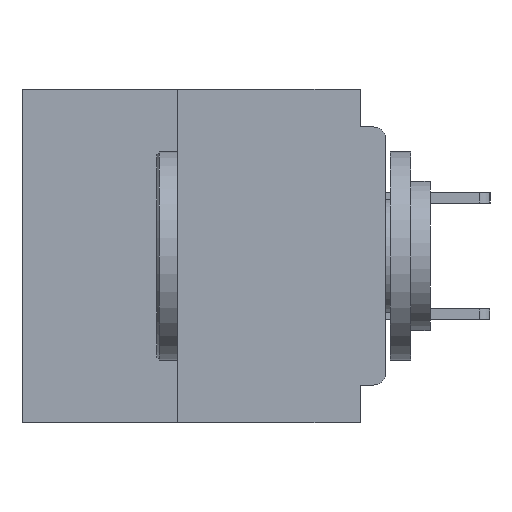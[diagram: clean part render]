
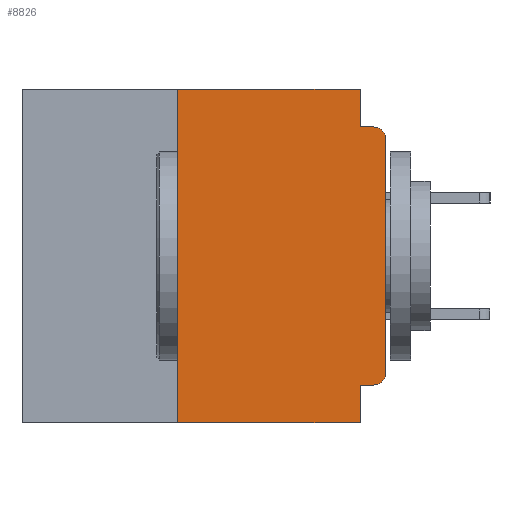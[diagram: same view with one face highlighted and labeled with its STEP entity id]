
A CAD part, left-side view. The second image highlights one B-rep face of the part: STEP entity #8826.
In plain terms, the highlighted planar face has unit normal (-1, 0, 0).
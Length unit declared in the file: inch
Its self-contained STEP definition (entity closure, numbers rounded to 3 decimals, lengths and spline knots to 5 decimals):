
#51 = VERTEX_POINT ( 'NONE', #12054 ) ;
#124 = LINE ( 'NONE', #33664, #1399 ) ;
#156 = FACE_OUTER_BOUND ( 'NONE', #11290, .T. ) ;
#342 = AXIS2_PLACEMENT_3D ( 'NONE', #40303, #16422, #44274 ) ;
#838 = CARTESIAN_POINT ( 'NONE',  ( 0., 0.437, 0. ) ) ;
#1216 = VERTEX_POINT ( 'NONE', #44864 ) ;
#1399 = VECTOR ( 'NONE', #13725, 39.37008 ) ;
#2683 = EDGE_CURVE ( 'NONE', #10931, #44653, #49319, .T. ) ;
#5147 = CARTESIAN_POINT ( 'NONE',  ( 0., 0., 0. ) ) ;
#6038 = VERTEX_POINT ( 'NONE', #50441 ) ;
#7062 = CARTESIAN_POINT ( 'NONE',  ( 0., 0.031, -0.355 ) ) ;
#7773 = CARTESIAN_POINT ( 'NONE',  ( 0., 0.031, -0.045 ) ) ;
#8325 = EDGE_CURVE ( 'NONE', #23445, #51, #45398, .T. ) ;
#8826 = ADVANCED_FACE ( 'NONE', ( #156 ), #36322, .F. ) ;
#9465 = CARTESIAN_POINT ( 'NONE',  ( 0., 0.031, -0.4 ) ) ;
#10931 = VERTEX_POINT ( 'NONE', #7062 ) ;
#11290 = EDGE_LOOP ( 'NONE', ( #17904, #48999, #14149, #24215, #12917, #45977, #40409, #33611, #34852, #19923 ) ) ;
#11738 = CARTESIAN_POINT ( 'NONE',  ( 0., 0.25, -0.4 ) ) ;
#12054 = CARTESIAN_POINT ( 'NONE',  ( 0., 0.015, -0.045 ) ) ;
#12917 = ORIENTED_EDGE ( 'NONE', *, *, #33629, .F. ) ;
#13236 = VECTOR ( 'NONE', #13382, 39.37008 ) ;
#13382 = DIRECTION ( 'NONE',  ( 0., 0., 1. ) ) ;
#13483 = CARTESIAN_POINT ( 'NONE',  ( 0., 0., -0.355 ) ) ;
#13725 = DIRECTION ( 'NONE',  ( 0., -1., 0. ) ) ;
#13757 = DIRECTION ( 'NONE',  ( 0., 0., -1. ) ) ;
#14149 = ORIENTED_EDGE ( 'NONE', *, *, #31255, .F. ) ;
#14887 = LINE ( 'NONE', #11738, #44169 ) ;
#15347 = LINE ( 'NONE', #48682, #50838 ) ;
#15582 = CARTESIAN_POINT ( 'NONE',  ( 0., 0., -0.06 ) ) ;
#16422 = DIRECTION ( 'NONE',  ( 1., 0., 0. ) ) ;
#16811 = CARTESIAN_POINT ( 'NONE',  ( 0., 0.25, -0.4 ) ) ;
#17904 = ORIENTED_EDGE ( 'NONE', *, *, #34433, .T. ) ;
#18618 = CIRCLE ( 'NONE', #23411, 0.015 ) ;
#19085 = VERTEX_POINT ( 'NONE', #39088 ) ;
#19464 = VECTOR ( 'NONE', #29627, 39.37008 ) ;
#19923 = ORIENTED_EDGE ( 'NONE', *, *, #20035, .T. ) ;
#20035 = EDGE_CURVE ( 'NONE', #19085, #1216, #18618, .T. ) ;
#20743 = LINE ( 'NONE', #13483, #19464 ) ;
#21124 = DIRECTION ( 'NONE',  ( 0., -1., 0. ) ) ;
#21280 = DIRECTION ( 'NONE',  ( 0., -1., 0. ) ) ;
#21284 = LINE ( 'NONE', #37686, #31848 ) ;
#21414 = VECTOR ( 'NONE', #35941, 39.37008 ) ;
#21623 = VERTEX_POINT ( 'NONE', #7773 ) ;
#21632 = DIRECTION ( 'NONE',  ( -1., 0., 0. ) ) ;
#22126 = CARTESIAN_POINT ( 'NONE',  ( 0., 0.015, -0.34 ) ) ;
#23411 = AXIS2_PLACEMENT_3D ( 'NONE', #22126, #49857, #26115 ) ;
#23445 = VERTEX_POINT ( 'NONE', #15582 ) ;
#23892 = DIRECTION ( 'NONE',  ( 0., 0., 1. ) ) ;
#24099 = AXIS2_PLACEMENT_3D ( 'NONE', #45369, #21632, #49335 ) ;
#24215 = ORIENTED_EDGE ( 'NONE', *, *, #29683, .F. ) ;
#26115 = DIRECTION ( 'NONE',  ( 0., 0., -1. ) ) ;
#26964 = EDGE_CURVE ( 'NONE', #19085, #10931, #20743, .T. ) ;
#28935 = VECTOR ( 'NONE', #21280, 39.37008 ) ;
#29627 = DIRECTION ( 'NONE',  ( 0., 1., 0. ) ) ;
#29683 = EDGE_CURVE ( 'NONE', #33683, #21623, #21284, .T. ) ;
#31255 = EDGE_CURVE ( 'NONE', #21623, #51, #124, .T. ) ;
#31848 = VECTOR ( 'NONE', #13757, 39.37008 ) ;
#32282 = VERTEX_POINT ( 'NONE', #16811 ) ;
#33611 = ORIENTED_EDGE ( 'NONE', *, *, #2683, .F. ) ;
#33629 = EDGE_CURVE ( 'NONE', #6038, #33683, #39476, .T. ) ;
#33664 = CARTESIAN_POINT ( 'NONE',  ( 0., 0., -0.045 ) ) ;
#33683 = VERTEX_POINT ( 'NONE', #41247 ) ;
#34433 = EDGE_CURVE ( 'NONE', #1216, #23445, #37008, .T. ) ;
#34852 = ORIENTED_EDGE ( 'NONE', *, *, #26964, .F. ) ;
#35941 = DIRECTION ( 'NONE',  ( 0., 0., -1. ) ) ;
#36322 = PLANE ( 'NONE',  #342 ) ;
#36370 = CARTESIAN_POINT ( 'NONE',  ( 0., 0.031, -0.4 ) ) ;
#37008 = LINE ( 'NONE', #5147, #13236 ) ;
#37686 = CARTESIAN_POINT ( 'NONE',  ( 0., 0.031, 0. ) ) ;
#39088 = CARTESIAN_POINT ( 'NONE',  ( 0., 0.015, -0.355 ) ) ;
#39476 = LINE ( 'NONE', #838, #28935 ) ;
#40303 = CARTESIAN_POINT ( 'NONE',  ( 0., 0.437, 0. ) ) ;
#40409 = ORIENTED_EDGE ( 'NONE', *, *, #48857, .T. ) ;
#41247 = CARTESIAN_POINT ( 'NONE',  ( 0., 0.031, 0. ) ) ;
#44169 = VECTOR ( 'NONE', #23892, 39.37008 ) ;
#44274 = DIRECTION ( 'NONE',  ( 0., 0., -1. ) ) ;
#44653 = VERTEX_POINT ( 'NONE', #9465 ) ;
#44864 = CARTESIAN_POINT ( 'NONE',  ( 0., 0., -0.34 ) ) ;
#45369 = CARTESIAN_POINT ( 'NONE',  ( 0., 0.015, -0.06 ) ) ;
#45398 = CIRCLE ( 'NONE', #24099, 0.015 ) ;
#45977 = ORIENTED_EDGE ( 'NONE', *, *, #47334, .F. ) ;
#47334 = EDGE_CURVE ( 'NONE', #32282, #6038, #14887, .T. ) ;
#48682 = CARTESIAN_POINT ( 'NONE',  ( 0., 0.437, -0.4 ) ) ;
#48857 = EDGE_CURVE ( 'NONE', #32282, #44653, #15347, .T. ) ;
#48999 = ORIENTED_EDGE ( 'NONE', *, *, #8325, .T. ) ;
#49319 = LINE ( 'NONE', #36370, #21414 ) ;
#49335 = DIRECTION ( 'NONE',  ( 0., 0., -1. ) ) ;
#49857 = DIRECTION ( 'NONE',  ( -1., 0., 0. ) ) ;
#50441 = CARTESIAN_POINT ( 'NONE',  ( 0., 0.25, 0. ) ) ;
#50838 = VECTOR ( 'NONE', #21124, 39.37008 ) ;
